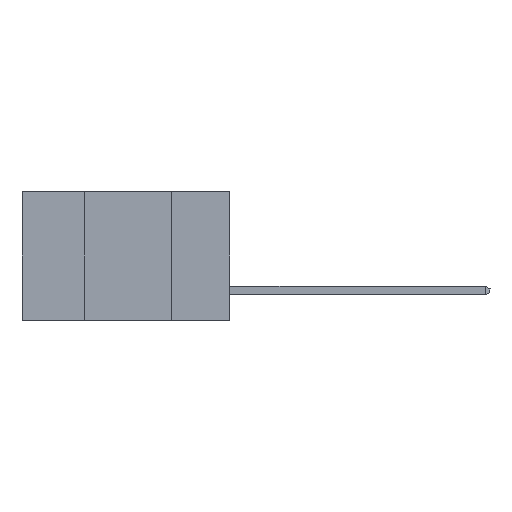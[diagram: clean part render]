
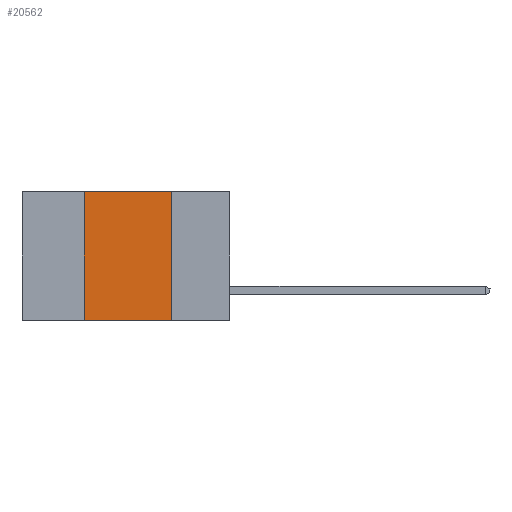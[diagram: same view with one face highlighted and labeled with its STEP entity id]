
A CAD part, left-side view. The second image highlights one B-rep face of the part: STEP entity #20562.
In plain terms, the highlighted planar face has unit normal (-1, 0, 0).
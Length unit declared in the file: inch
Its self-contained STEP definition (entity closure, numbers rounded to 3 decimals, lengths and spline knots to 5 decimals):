
#492 = VECTOR ( 'NONE', #3287, 39.37008 ) ;
#575 = LINE ( 'NONE', #6940, #16649 ) ;
#1876 = CARTESIAN_POINT ( 'NONE',  ( 0., 0.6, 0. ) ) ;
#2528 = CARTESIAN_POINT ( 'NONE',  ( 0., 0.42, -0.37 ) ) ;
#2633 = DIRECTION ( 'NONE',  ( 0., 0., 1. ) ) ;
#3174 = CARTESIAN_POINT ( 'NONE',  ( 0., 0.17, -0.37 ) ) ;
#3287 = DIRECTION ( 'NONE',  ( 0., -1., 0. ) ) ;
#3391 = PLANE ( 'NONE',  #21238 ) ;
#4465 = LINE ( 'NONE', #2528, #18665 ) ;
#5083 = CARTESIAN_POINT ( 'NONE',  ( 0., 0.17, 0. ) ) ;
#5217 = DIRECTION ( 'NONE',  ( 0., 0., -1. ) ) ;
#5338 = VERTEX_POINT ( 'NONE', #13670 ) ;
#6069 = VERTEX_POINT ( 'NONE', #5083 ) ;
#6940 = CARTESIAN_POINT ( 'NONE',  ( 0., 0.17, -0.37 ) ) ;
#7687 = VECTOR ( 'NONE', #9711, 39.37008 ) ;
#8459 = LINE ( 'NONE', #1876, #492 ) ;
#8674 = FACE_OUTER_BOUND ( 'NONE', #16133, .T. ) ;
#9711 = DIRECTION ( 'NONE',  ( 0., -1., 0. ) ) ;
#10475 = ORIENTED_EDGE ( 'NONE', *, *, #12935, .F. ) ;
#12935 = EDGE_CURVE ( 'NONE', #16843, #5338, #4465, .T. ) ;
#13572 = CARTESIAN_POINT ( 'NONE',  ( 0., 0.42, -0.37 ) ) ;
#13670 = CARTESIAN_POINT ( 'NONE',  ( 0., 0.42, 0. ) ) ;
#15257 = DIRECTION ( 'NONE',  ( 1., 0., 0. ) ) ;
#16065 = LINE ( 'NONE', #19289, #7687 ) ;
#16084 = VERTEX_POINT ( 'NONE', #3174 ) ;
#16133 = EDGE_LOOP ( 'NONE', ( #17961, #19424, #10475, #16624 ) ) ;
#16327 = EDGE_CURVE ( 'NONE', #6069, #16084, #575, .T. ) ;
#16411 = EDGE_CURVE ( 'NONE', #16843, #16084, #16065, .T. ) ;
#16624 = ORIENTED_EDGE ( 'NONE', *, *, #16411, .T. ) ;
#16640 = DIRECTION ( 'NONE',  ( 0., 0., -1. ) ) ;
#16649 = VECTOR ( 'NONE', #5217, 39.37008 ) ;
#16843 = VERTEX_POINT ( 'NONE', #13572 ) ;
#17458 = EDGE_CURVE ( 'NONE', #5338, #6069, #8459, .T. ) ;
#17961 = ORIENTED_EDGE ( 'NONE', *, *, #16327, .F. ) ;
#18469 = CARTESIAN_POINT ( 'NONE',  ( 0., 0.6, 0. ) ) ;
#18665 = VECTOR ( 'NONE', #2633, 39.37008 ) ;
#19289 = CARTESIAN_POINT ( 'NONE',  ( 0., 0.6, -0.37 ) ) ;
#19424 = ORIENTED_EDGE ( 'NONE', *, *, #17458, .F. ) ;
#20562 = ADVANCED_FACE ( 'NONE', ( #8674 ), #3391, .F. ) ;
#21238 = AXIS2_PLACEMENT_3D ( 'NONE', #18469, #15257, #16640 ) ;
